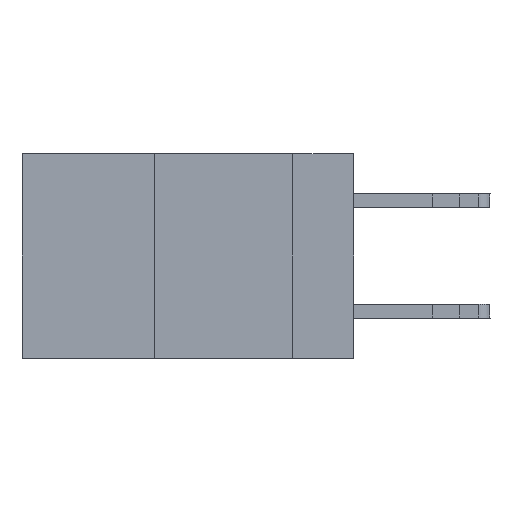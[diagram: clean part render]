
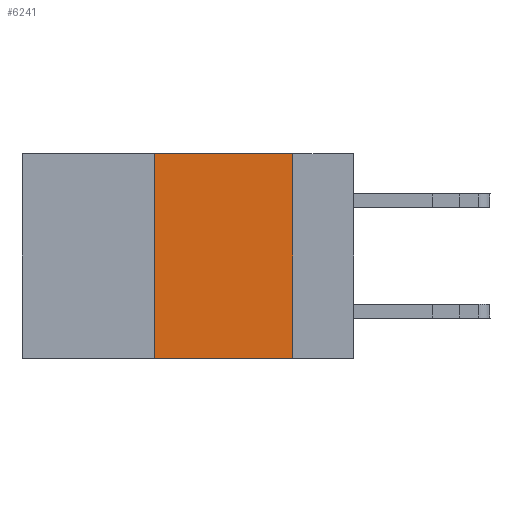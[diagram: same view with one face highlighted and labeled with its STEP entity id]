
A CAD part, left-side view. The second image highlights one B-rep face of the part: STEP entity #6241.
In plain terms, the highlighted planar face has unit normal (-1, 0, 0).
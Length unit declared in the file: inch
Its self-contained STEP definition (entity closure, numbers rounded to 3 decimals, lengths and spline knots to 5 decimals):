
#978 = EDGE_CURVE ( 'NONE', #16014, #15407, #14229, .T. ) ;
#1124 = CARTESIAN_POINT ( 'NONE',  ( 0., 0.6, -0.37 ) ) ;
#2338 = EDGE_LOOP ( 'NONE', ( #6898, #4734, #21974, #6908 ) ) ;
#4431 = LINE ( 'NONE', #4543, #8102 ) ;
#4543 = CARTESIAN_POINT ( 'NONE',  ( 0., 0.36, 0. ) ) ;
#4614 = DIRECTION ( 'NONE',  ( 0., -1., 0. ) ) ;
#4734 = ORIENTED_EDGE ( 'NONE', *, *, #6097, .F. ) ;
#4736 = LINE ( 'NONE', #20728, #23581 ) ;
#6038 = LINE ( 'NONE', #8198, #10228 ) ;
#6097 = EDGE_CURVE ( 'NONE', #22224, #11809, #4736, .T. ) ;
#6241 = ADVANCED_FACE ( 'NONE', ( #21422 ), #21787, .F. ) ;
#6898 = ORIENTED_EDGE ( 'NONE', *, *, #8989, .F. ) ;
#6908 = ORIENTED_EDGE ( 'NONE', *, *, #978, .T. ) ;
#8102 = VECTOR ( 'NONE', #19209, 39.37008 ) ;
#8198 = CARTESIAN_POINT ( 'NONE',  ( 0., 0.11, 0. ) ) ;
#8955 = DIRECTION ( 'NONE',  ( 1., 0., 0. ) ) ;
#8989 = EDGE_CURVE ( 'NONE', #11809, #15407, #6038, .T. ) ;
#9298 = CARTESIAN_POINT ( 'NONE',  ( 0., 0.36, 0. ) ) ;
#10228 = VECTOR ( 'NONE', #19126, 39.37008 ) ;
#11672 = CARTESIAN_POINT ( 'NONE',  ( 0., 0.36, -0.37 ) ) ;
#11809 = VERTEX_POINT ( 'NONE', #19517 ) ;
#12309 = DIRECTION ( 'NONE',  ( 0., 0., -1. ) ) ;
#14229 = LINE ( 'NONE', #1124, #17885 ) ;
#14484 = CARTESIAN_POINT ( 'NONE',  ( 0., 0.6, 0. ) ) ;
#14629 = EDGE_CURVE ( 'NONE', #16014, #22224, #4431, .T. ) ;
#15407 = VERTEX_POINT ( 'NONE', #20474 ) ;
#16014 = VERTEX_POINT ( 'NONE', #11672 ) ;
#17885 = VECTOR ( 'NONE', #21525, 39.37008 ) ;
#19126 = DIRECTION ( 'NONE',  ( 0., 0., -1. ) ) ;
#19209 = DIRECTION ( 'NONE',  ( 0., 0., 1. ) ) ;
#19384 = AXIS2_PLACEMENT_3D ( 'NONE', #14484, #8955, #12309 ) ;
#19517 = CARTESIAN_POINT ( 'NONE',  ( 0., 0.11, 0. ) ) ;
#20474 = CARTESIAN_POINT ( 'NONE',  ( 0., 0.11, -0.37 ) ) ;
#20728 = CARTESIAN_POINT ( 'NONE',  ( 0., 0.6, 0. ) ) ;
#21422 = FACE_OUTER_BOUND ( 'NONE', #2338, .T. ) ;
#21525 = DIRECTION ( 'NONE',  ( 0., -1., 0. ) ) ;
#21787 = PLANE ( 'NONE',  #19384 ) ;
#21974 = ORIENTED_EDGE ( 'NONE', *, *, #14629, .F. ) ;
#22224 = VERTEX_POINT ( 'NONE', #9298 ) ;
#23581 = VECTOR ( 'NONE', #4614, 39.37008 ) ;
